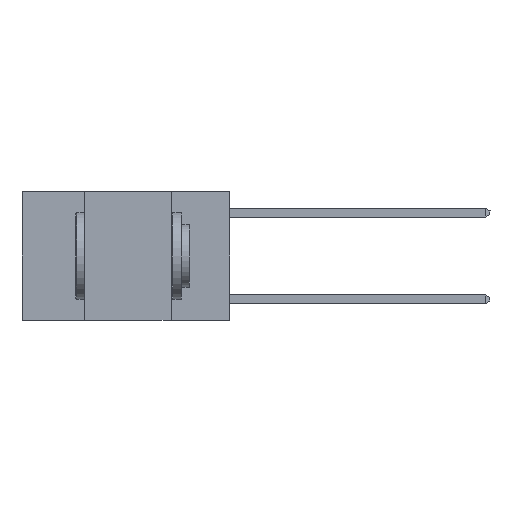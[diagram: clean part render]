
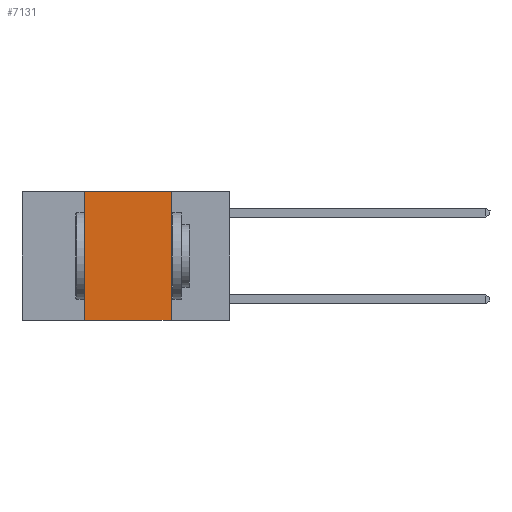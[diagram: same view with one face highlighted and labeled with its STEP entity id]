
A CAD part, left-side view. The second image highlights one B-rep face of the part: STEP entity #7131.
In plain terms, the highlighted planar face has unit normal (-1, 0, 0).
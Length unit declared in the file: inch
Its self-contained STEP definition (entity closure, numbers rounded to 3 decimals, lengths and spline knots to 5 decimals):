
#273 = VECTOR ( 'NONE', #20686, 39.37008 ) ;
#777 = VERTEX_POINT ( 'NONE', #15120 ) ;
#1451 = EDGE_CURVE ( 'NONE', #14083, #12276, #2675, .T. ) ;
#1955 = DIRECTION ( 'NONE',  ( 0., -1., 0. ) ) ;
#2431 = ORIENTED_EDGE ( 'NONE', *, *, #1451, .T. ) ;
#2675 = LINE ( 'NONE', #12492, #16744 ) ;
#4328 = DIRECTION ( 'NONE',  ( 0., -1., 0. ) ) ;
#4660 = VECTOR ( 'NONE', #1955, 39.37008 ) ;
#4838 = DIRECTION ( 'NONE',  ( 1., 0., 0. ) ) ;
#4978 = ORIENTED_EDGE ( 'NONE', *, *, #5254, .F. ) ;
#5123 = CARTESIAN_POINT ( 'NONE',  ( 0., 0.6, 0. ) ) ;
#5254 = EDGE_CURVE ( 'NONE', #777, #12276, #21113, .T. ) ;
#6571 = DIRECTION ( 'NONE',  ( 0., 0., -1. ) ) ;
#6768 = VECTOR ( 'NONE', #13189, 39.37008 ) ;
#7131 = ADVANCED_FACE ( 'NONE', ( #11585 ), #11687, .F. ) ;
#7680 = VERTEX_POINT ( 'NONE', #8516 ) ;
#8312 = CARTESIAN_POINT ( 'NONE',  ( 0., 0.42, 0. ) ) ;
#8516 = CARTESIAN_POINT ( 'NONE',  ( 0., 0.42, 0. ) ) ;
#9429 = ORIENTED_EDGE ( 'NONE', *, *, #16134, .F. ) ;
#10747 = CARTESIAN_POINT ( 'NONE',  ( 0., 0.17, 0. ) ) ;
#11585 = FACE_OUTER_BOUND ( 'NONE', #16823, .T. ) ;
#11687 = PLANE ( 'NONE',  #18626 ) ;
#11980 = CARTESIAN_POINT ( 'NONE',  ( 0., 0.17, -0.37 ) ) ;
#12276 = VERTEX_POINT ( 'NONE', #11980 ) ;
#12492 = CARTESIAN_POINT ( 'NONE',  ( 0., 0.6, -0.37 ) ) ;
#13189 = DIRECTION ( 'NONE',  ( 0., 0., 1. ) ) ;
#14083 = VERTEX_POINT ( 'NONE', #16630 ) ;
#14123 = EDGE_CURVE ( 'NONE', #14083, #7680, #18027, .T. ) ;
#15120 = CARTESIAN_POINT ( 'NONE',  ( 0., 0.17, 0. ) ) ;
#15199 = LINE ( 'NONE', #5123, #4660 ) ;
#16134 = EDGE_CURVE ( 'NONE', #7680, #777, #15199, .T. ) ;
#16534 = CARTESIAN_POINT ( 'NONE',  ( 0., 0.6, 0. ) ) ;
#16630 = CARTESIAN_POINT ( 'NONE',  ( 0., 0.42, -0.37 ) ) ;
#16744 = VECTOR ( 'NONE', #4328, 39.37008 ) ;
#16823 = EDGE_LOOP ( 'NONE', ( #4978, #9429, #18912, #2431 ) ) ;
#18027 = LINE ( 'NONE', #8312, #6768 ) ;
#18626 = AXIS2_PLACEMENT_3D ( 'NONE', #16534, #4838, #6571 ) ;
#18912 = ORIENTED_EDGE ( 'NONE', *, *, #14123, .F. ) ;
#20686 = DIRECTION ( 'NONE',  ( 0., 0., -1. ) ) ;
#21113 = LINE ( 'NONE', #10747, #273 ) ;
